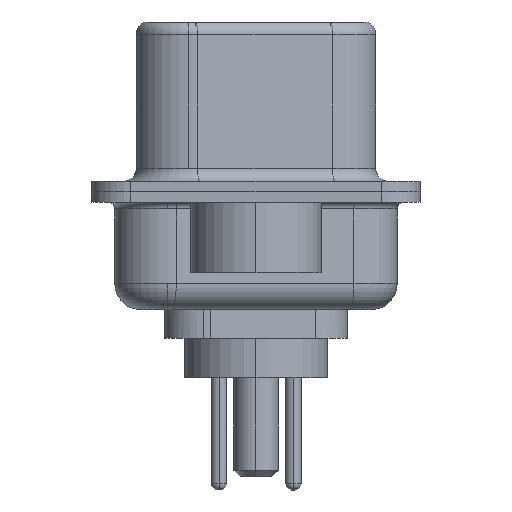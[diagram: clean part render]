
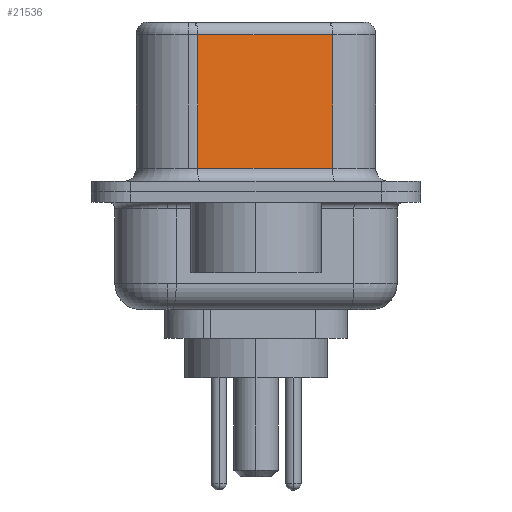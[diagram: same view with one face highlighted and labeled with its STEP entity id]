
A CAD part, left-side view. The second image highlights one B-rep face of the part: STEP entity #21536.
In plain terms, the highlighted planar face has unit normal (-0.985, -0.174, 0).
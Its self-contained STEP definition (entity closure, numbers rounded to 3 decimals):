
#803 = VERTEX_POINT ( 'NONE', #12631 ) ;
#1442 = LINE ( 'NONE', #2059, #22850 ) ;
#1908 = DIRECTION ( 'NONE',  ( 0., 0., -1. ) ) ;
#2059 = CARTESIAN_POINT ( 'NONE',  ( 3.67, 2.233, 6.52 ) ) ;
#2526 = VECTOR ( 'NONE', #8382, 1000. ) ;
#2866 = EDGE_CURVE ( 'NONE', #21554, #803, #13035, .T. ) ;
#2938 = FACE_OUTER_BOUND ( 'NONE', #10905, .T. ) ;
#6007 = VECTOR ( 'NONE', #1908, 1000. ) ;
#8240 = LINE ( 'NONE', #9245, #9493 ) ;
#8382 = DIRECTION ( 'NONE',  ( -0.174, 0.985, 0. ) ) ;
#8568 = CARTESIAN_POINT ( 'NONE',  ( 4.58, -2.927, 6.02 ) ) ;
#9245 = CARTESIAN_POINT ( 'NONE',  ( 4.58, -2.927, 0.9 ) ) ;
#9493 = VECTOR ( 'NONE', #22752, 1000. ) ;
#10036 = ORIENTED_EDGE ( 'NONE', *, *, #21427, .F. ) ;
#10045 = VERTEX_POINT ( 'NONE', #17400 ) ;
#10266 = DIRECTION ( 'NONE',  ( -0.174, 0.985, 0. ) ) ;
#10905 = EDGE_LOOP ( 'NONE', ( #10036, #11606, #18843, #14861 ) ) ;
#11606 = ORIENTED_EDGE ( 'NONE', *, *, #2866, .T. ) ;
#12127 = PLANE ( 'NONE',  #14556 ) ;
#12631 = CARTESIAN_POINT ( 'NONE',  ( 3.67, 2.233, 6.02 ) ) ;
#12750 = EDGE_CURVE ( 'NONE', #803, #14072, #1442, .T. ) ;
#13035 = LINE ( 'NONE', #8568, #2526 ) ;
#13892 = DIRECTION ( 'NONE',  ( 0., 0., -1. ) ) ;
#14072 = VERTEX_POINT ( 'NONE', #22417 ) ;
#14198 = EDGE_CURVE ( 'NONE', #14072, #10045, #8240, .T. ) ;
#14556 = AXIS2_PLACEMENT_3D ( 'NONE', #16005, #21787, #10266 ) ;
#14861 = ORIENTED_EDGE ( 'NONE', *, *, #14198, .T. ) ;
#15661 = CARTESIAN_POINT ( 'NONE',  ( 4.58, -2.927, 6.52 ) ) ;
#15784 = LINE ( 'NONE', #15661, #6007 ) ;
#16005 = CARTESIAN_POINT ( 'NONE',  ( 4.58, -2.927, 6.52 ) ) ;
#17400 = CARTESIAN_POINT ( 'NONE',  ( 4.58, -2.927, 0.9 ) ) ;
#18843 = ORIENTED_EDGE ( 'NONE', *, *, #12750, .T. ) ;
#21427 = EDGE_CURVE ( 'NONE', #21554, #10045, #15784, .T. ) ;
#21536 = ADVANCED_FACE ( 'NONE', ( #2938 ), #12127, .F. ) ;
#21554 = VERTEX_POINT ( 'NONE', #23731 ) ;
#21787 = DIRECTION ( 'NONE',  ( 0.985, 0.174, 0. ) ) ;
#22417 = CARTESIAN_POINT ( 'NONE',  ( 3.67, 2.233, 0.9 ) ) ;
#22752 = DIRECTION ( 'NONE',  ( 0.174, -0.985, 0. ) ) ;
#22850 = VECTOR ( 'NONE', #13892, 1000. ) ;
#23731 = CARTESIAN_POINT ( 'NONE',  ( 4.58, -2.927, 6.02 ) ) ;
